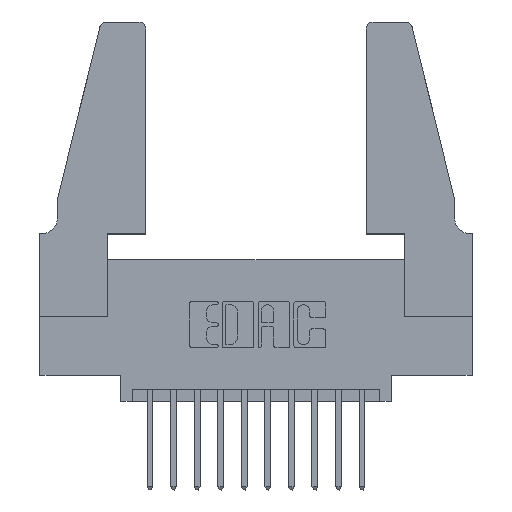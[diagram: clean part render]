
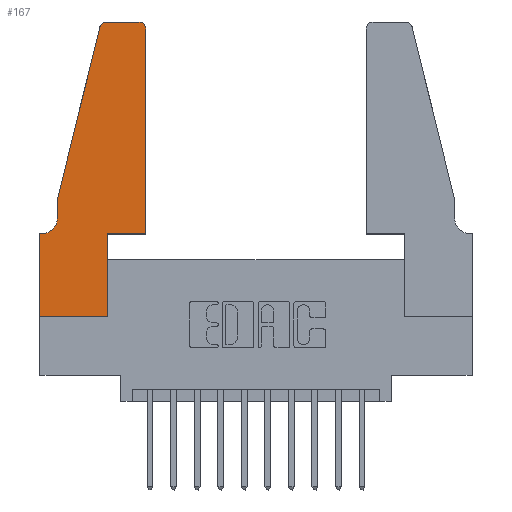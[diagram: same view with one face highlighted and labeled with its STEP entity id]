
A CAD part, top view. The second image highlights one B-rep face of the part: STEP entity #167.
In plain terms, the highlighted planar face has unit normal (0, 0, 1).
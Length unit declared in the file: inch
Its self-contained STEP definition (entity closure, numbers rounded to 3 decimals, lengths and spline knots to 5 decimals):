
#112 = LINE ( 'NONE', #5197, #11831 ) ;
#167 = ADVANCED_FACE ( 'NONE', ( #2499 ), #1531, .T. ) ;
#230 = CARTESIAN_POINT ( 'NONE',  ( 0.4205, 1.22, 0.37 ) ) ;
#237 = DIRECTION ( 'NONE',  ( 0., -1., 0. ) ) ;
#277 = LINE ( 'NONE', #10563, #12598 ) ;
#492 = VERTEX_POINT ( 'NONE', #6872 ) ;
#572 = ORIENTED_EDGE ( 'NONE', *, *, #10118, .T. ) ;
#717 = VERTEX_POINT ( 'NONE', #6215 ) ;
#1052 = EDGE_CURVE ( 'NONE', #3553, #8511, #12689, .T. ) ;
#1118 = DIRECTION ( 'NONE',  ( 1., 0., 0. ) ) ;
#1445 = DIRECTION ( 'NONE',  ( 0., 0., 1. ) ) ;
#1463 = DIRECTION ( 'NONE',  ( 1., 0., 0. ) ) ;
#1474 = DIRECTION ( 'NONE',  ( 0., 0., 1. ) ) ;
#1486 = CARTESIAN_POINT ( 'NONE',  ( 0.4205, 1.25, 0.37 ) ) ;
#1531 = PLANE ( 'NONE',  #7396 ) ;
#1584 = CARTESIAN_POINT ( 'NONE',  ( 0., 0.35, 0.37 ) ) ;
#1702 = EDGE_LOOP ( 'NONE', ( #3402, #9727, #12282, #7653, #14080, #10640, #572, #7539, #10989, #5008, #9806, #4153 ) ) ;
#1729 = LINE ( 'NONE', #8745, #7462 ) ;
#1757 = DIRECTION ( 'NONE',  ( -0.239, -0.971, 0. ) ) ;
#1908 = CARTESIAN_POINT ( 'NONE',  ( 0.2605, 1.25, 0.37 ) ) ;
#2499 = FACE_OUTER_BOUND ( 'NONE', #1702, .T. ) ;
#2520 = CARTESIAN_POINT ( 'NONE',  ( 0.25487, 1.22718, 0.37 ) ) ;
#2623 = DIRECTION ( 'NONE',  ( 0., 1., 0. ) ) ;
#2830 = CIRCLE ( 'NONE', #9859, 0.03 ) ;
#2903 = VECTOR ( 'NONE', #237, 39.37008 ) ;
#2913 = CARTESIAN_POINT ( 'NONE',  ( 0.4505, 0.35, 0.37 ) ) ;
#3112 = DIRECTION ( 'NONE',  ( -1., 0., 0. ) ) ;
#3154 = DIRECTION ( 'NONE',  ( 1., 0., 0. ) ) ;
#3172 = VERTEX_POINT ( 'NONE', #2913 ) ;
#3402 = ORIENTED_EDGE ( 'NONE', *, *, #10329, .T. ) ;
#3553 = VERTEX_POINT ( 'NONE', #7944 ) ;
#3949 = DIRECTION ( 'NONE',  ( 0., -1., 0. ) ) ;
#4017 = AXIS2_PLACEMENT_3D ( 'NONE', #8290, #1445, #9378 ) ;
#4120 = VERTEX_POINT ( 'NONE', #1486 ) ;
#4153 = ORIENTED_EDGE ( 'NONE', *, *, #7925, .T. ) ;
#4303 = DIRECTION ( 'NONE',  ( 1., 0., 0. ) ) ;
#4341 = AXIS2_PLACEMENT_3D ( 'NONE', #9393, #9390, #10657 ) ;
#4487 = LINE ( 'NONE', #4904, #13151 ) ;
#4904 = CARTESIAN_POINT ( 'NONE',  ( 0.4505, 0.35, 0.37 ) ) ;
#5008 = ORIENTED_EDGE ( 'NONE', *, *, #7112, .T. ) ;
#5040 = EDGE_CURVE ( 'NONE', #717, #3553, #8541, .T. ) ;
#5172 = LINE ( 'NONE', #9353, #5536 ) ;
#5197 = CARTESIAN_POINT ( 'NONE',  ( 0.0755, 0.35, 0.37 ) ) ;
#5536 = VECTOR ( 'NONE', #2623, 39.37008 ) ;
#5770 = VERTEX_POINT ( 'NONE', #8545 ) ;
#6215 = CARTESIAN_POINT ( 'NONE',  ( 0.0755, 0.5, 0.37 ) ) ;
#6556 = CARTESIAN_POINT ( 'NONE',  ( 0., 0.35, 0.37 ) ) ;
#6577 = VECTOR ( 'NONE', #1757, 39.37008 ) ;
#6872 = CARTESIAN_POINT ( 'NONE',  ( 0.2865, 0., 0.37 ) ) ;
#7032 = LINE ( 'NONE', #1908, #13136 ) ;
#7112 = EDGE_CURVE ( 'NONE', #10136, #3172, #1729, .T. ) ;
#7396 = AXIS2_PLACEMENT_3D ( 'NONE', #1584, #1474, #1118 ) ;
#7462 = VECTOR ( 'NONE', #3154, 39.37008 ) ;
#7539 = ORIENTED_EDGE ( 'NONE', *, *, #9314, .T. ) ;
#7653 = ORIENTED_EDGE ( 'NONE', *, *, #5040, .T. ) ;
#7925 = EDGE_CURVE ( 'NONE', #9329, #4120, #2830, .T. ) ;
#7944 = CARTESIAN_POINT ( 'NONE',  ( 0.0755, 0.42, 0.37 ) ) ;
#8104 = DIRECTION ( 'NONE',  ( 0., 1., 0. ) ) ;
#8176 = VERTEX_POINT ( 'NONE', #6556 ) ;
#8290 = CARTESIAN_POINT ( 'NONE',  ( 0.284, 1.22, 0.37 ) ) ;
#8305 = DIRECTION ( 'NONE',  ( 0., 0., 1. ) ) ;
#8431 = VECTOR ( 'NONE', #4303, 39.37008 ) ;
#8511 = VERTEX_POINT ( 'NONE', #9478 ) ;
#8541 = LINE ( 'NONE', #11599, #2903 ) ;
#8545 = CARTESIAN_POINT ( 'NONE',  ( 0., 0., 0.37 ) ) ;
#8745 = CARTESIAN_POINT ( 'NONE',  ( 0.4505, 0.35, 0.37 ) ) ;
#9215 = EDGE_CURVE ( 'NONE', #9650, #717, #9447, .T. ) ;
#9314 = EDGE_CURVE ( 'NONE', #5770, #492, #10970, .T. ) ;
#9329 = VERTEX_POINT ( 'NONE', #14076 ) ;
#9353 = CARTESIAN_POINT ( 'NONE',  ( 0.2865, 0.35, 0.37 ) ) ;
#9378 = DIRECTION ( 'NONE',  ( 1., 0., 0. ) ) ;
#9390 = DIRECTION ( 'NONE',  ( 0., 0., -1. ) ) ;
#9393 = CARTESIAN_POINT ( 'NONE',  ( 0.0055, 0.42, 0.37 ) ) ;
#9447 = LINE ( 'NONE', #9616, #6577 ) ;
#9462 = CARTESIAN_POINT ( 'NONE',  ( 0.2865, 0.35, 0.37 ) ) ;
#9478 = CARTESIAN_POINT ( 'NONE',  ( 0.0055, 0.35, 0.37 ) ) ;
#9616 = CARTESIAN_POINT ( 'NONE',  ( 0.0755, 0.5, 0.37 ) ) ;
#9650 = VERTEX_POINT ( 'NONE', #2520 ) ;
#9727 = ORIENTED_EDGE ( 'NONE', *, *, #13618, .T. ) ;
#9774 = CIRCLE ( 'NONE', #4017, 0.03 ) ;
#9806 = ORIENTED_EDGE ( 'NONE', *, *, #11743, .T. ) ;
#9859 = AXIS2_PLACEMENT_3D ( 'NONE', #230, #8305, #1463 ) ;
#9997 = VERTEX_POINT ( 'NONE', #13086 ) ;
#10118 = EDGE_CURVE ( 'NONE', #8176, #5770, #277, .T. ) ;
#10136 = VERTEX_POINT ( 'NONE', #9462 ) ;
#10329 = EDGE_CURVE ( 'NONE', #4120, #9997, #7032, .T. ) ;
#10563 = CARTESIAN_POINT ( 'NONE',  ( 0., 0., 0.37 ) ) ;
#10640 = ORIENTED_EDGE ( 'NONE', *, *, #12612, .T. ) ;
#10657 = DIRECTION ( 'NONE',  ( -1., 0., 0. ) ) ;
#10680 = DIRECTION ( 'NONE',  ( -1., 0., 0. ) ) ;
#10883 = CARTESIAN_POINT ( 'NONE',  ( 0., 0., 0.37 ) ) ;
#10970 = LINE ( 'NONE', #10883, #8431 ) ;
#10989 = ORIENTED_EDGE ( 'NONE', *, *, #12482, .T. ) ;
#11599 = CARTESIAN_POINT ( 'NONE',  ( 0.0755, 0.5, 0.37 ) ) ;
#11743 = EDGE_CURVE ( 'NONE', #3172, #9329, #4487, .T. ) ;
#11831 = VECTOR ( 'NONE', #10680, 39.37008 ) ;
#12282 = ORIENTED_EDGE ( 'NONE', *, *, #9215, .T. ) ;
#12482 = EDGE_CURVE ( 'NONE', #492, #10136, #5172, .T. ) ;
#12598 = VECTOR ( 'NONE', #3949, 39.37008 ) ;
#12612 = EDGE_CURVE ( 'NONE', #8511, #8176, #112, .T. ) ;
#12689 = CIRCLE ( 'NONE', #4341, 0.07 ) ;
#13086 = CARTESIAN_POINT ( 'NONE',  ( 0.284, 1.25, 0.37 ) ) ;
#13136 = VECTOR ( 'NONE', #3112, 39.37008 ) ;
#13151 = VECTOR ( 'NONE', #8104, 39.37008 ) ;
#13618 = EDGE_CURVE ( 'NONE', #9997, #9650, #9774, .T. ) ;
#14076 = CARTESIAN_POINT ( 'NONE',  ( 0.4505, 1.22, 0.37 ) ) ;
#14080 = ORIENTED_EDGE ( 'NONE', *, *, #1052, .T. ) ;
